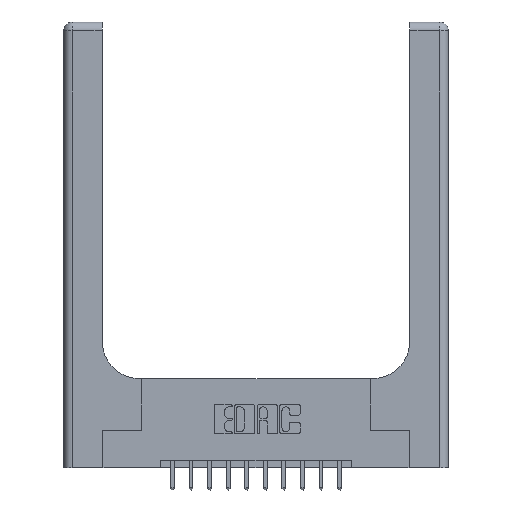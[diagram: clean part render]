
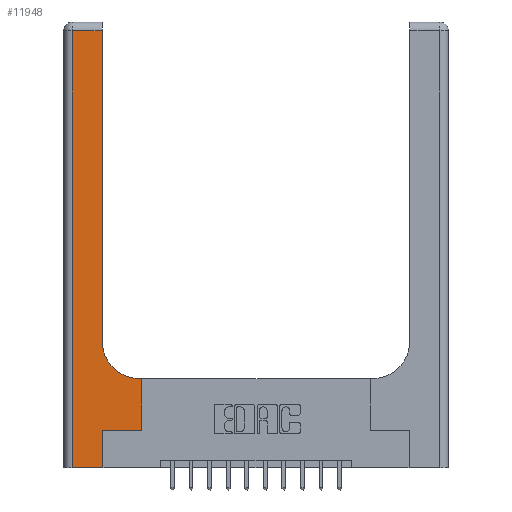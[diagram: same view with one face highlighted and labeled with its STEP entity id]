
A CAD part, top view. The second image highlights one B-rep face of the part: STEP entity #11948.
In plain terms, the highlighted planar face has unit normal (0, 0, 1).
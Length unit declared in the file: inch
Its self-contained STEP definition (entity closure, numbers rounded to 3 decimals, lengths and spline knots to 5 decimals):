
#190 = DIRECTION ( 'NONE',  ( -1., 0., 0. ) ) ;
#330 = VERTEX_POINT ( 'NONE', #12840 ) ;
#437 = CARTESIAN_POINT ( 'NONE',  ( 0.26, 0.6, 0.37 ) ) ;
#578 = EDGE_LOOP ( 'NONE', ( #8681, #5691, #9644, #4940, #738, #8904, #10867, #3484, #5365 ) ) ;
#738 = ORIENTED_EDGE ( 'NONE', *, *, #3867, .T. ) ;
#1101 = EDGE_CURVE ( 'NONE', #2566, #6404, #11632, .T. ) ;
#1329 = DIRECTION ( 'NONE',  ( 1., 0., 0. ) ) ;
#1360 = VERTEX_POINT ( 'NONE', #10355 ) ;
#1429 = CARTESIAN_POINT ( 'NONE',  ( 0.51, 0.85, 0.37 ) ) ;
#2566 = VERTEX_POINT ( 'NONE', #7742 ) ;
#2637 = VECTOR ( 'NONE', #8583, 39.37008 ) ;
#2664 = LINE ( 'NONE', #5162, #10751 ) ;
#2748 = AXIS2_PLACEMENT_3D ( 'NONE', #7198, #4822, #4665 ) ;
#2756 = DIRECTION ( 'NONE',  ( 1., 0., 0. ) ) ;
#2799 = DIRECTION ( 'NONE',  ( 0., 1., 0. ) ) ;
#2901 = DIRECTION ( 'NONE',  ( -1., 0., 0. ) ) ;
#3183 = CARTESIAN_POINT ( 'NONE',  ( 0.51, 0.6, 0.37 ) ) ;
#3458 = AXIS2_PLACEMENT_3D ( 'NONE', #1429, #14357, #2756 ) ;
#3475 = CARTESIAN_POINT ( 'NONE',  ( 0.26, 3., 0.37 ) ) ;
#3484 = ORIENTED_EDGE ( 'NONE', *, *, #1101, .T. ) ;
#3773 = CARTESIAN_POINT ( 'NONE',  ( 0.06, 3., 0.37 ) ) ;
#3837 = VECTOR ( 'NONE', #2901, 39.37008 ) ;
#3867 = EDGE_CURVE ( 'NONE', #11664, #1360, #13060, .T. ) ;
#4095 = VERTEX_POINT ( 'NONE', #4532 ) ;
#4496 = VECTOR ( 'NONE', #2799, 39.37008 ) ;
#4532 = CARTESIAN_POINT ( 'NONE',  ( 0.06, 2.94, 0.37 ) ) ;
#4665 = DIRECTION ( 'NONE',  ( -1., 0., 0. ) ) ;
#4822 = DIRECTION ( 'NONE',  ( 0., 0., -1. ) ) ;
#4940 = ORIENTED_EDGE ( 'NONE', *, *, #7980, .T. ) ;
#5162 = CARTESIAN_POINT ( 'NONE',  ( 0.265, 0.25, 0.37 ) ) ;
#5365 = ORIENTED_EDGE ( 'NONE', *, *, #6035, .T. ) ;
#5516 = EDGE_CURVE ( 'NONE', #4095, #8797, #15300, .T. ) ;
#5691 = ORIENTED_EDGE ( 'NONE', *, *, #15255, .T. ) ;
#5977 = VERTEX_POINT ( 'NONE', #10213 ) ;
#6035 = EDGE_CURVE ( 'NONE', #6404, #5977, #11730, .T. ) ;
#6404 = VERTEX_POINT ( 'NONE', #3183 ) ;
#6464 = VERTEX_POINT ( 'NONE', #8541 ) ;
#6630 = CARTESIAN_POINT ( 'NONE',  ( 0.528, 0.25, 0.37 ) ) ;
#7174 = VECTOR ( 'NONE', #1329, 39.37008 ) ;
#7198 = CARTESIAN_POINT ( 'NONE',  ( 0., 3., 0.37 ) ) ;
#7742 = CARTESIAN_POINT ( 'NONE',  ( 0.528, 0.6, 0.37 ) ) ;
#7810 = VECTOR ( 'NONE', #190, 39.37008 ) ;
#7980 = EDGE_CURVE ( 'NONE', #8797, #11664, #10191, .T. ) ;
#8384 = EDGE_CURVE ( 'NONE', #5977, #330, #11251, .T. ) ;
#8482 = EDGE_CURVE ( 'NONE', #6464, #2566, #9910, .T. ) ;
#8531 = PLANE ( 'NONE',  #2748 ) ;
#8541 = CARTESIAN_POINT ( 'NONE',  ( 0.528, 0.25, 0.37 ) ) ;
#8583 = DIRECTION ( 'NONE',  ( 0., 1., 0. ) ) ;
#8681 = ORIENTED_EDGE ( 'NONE', *, *, #8384, .T. ) ;
#8797 = VERTEX_POINT ( 'NONE', #11621 ) ;
#8904 = ORIENTED_EDGE ( 'NONE', *, *, #13293, .T. ) ;
#9644 = ORIENTED_EDGE ( 'NONE', *, *, #5516, .T. ) ;
#9910 = LINE ( 'NONE', #6630, #12240 ) ;
#10191 = LINE ( 'NONE', #15009, #7174 ) ;
#10213 = CARTESIAN_POINT ( 'NONE',  ( 0.26, 0.85, 0.37 ) ) ;
#10355 = CARTESIAN_POINT ( 'NONE',  ( 0.265, 0.25, 0.37 ) ) ;
#10568 = CARTESIAN_POINT ( 'NONE',  ( 0.265, 0., 0.37 ) ) ;
#10751 = VECTOR ( 'NONE', #11609, 39.37008 ) ;
#10867 = ORIENTED_EDGE ( 'NONE', *, *, #8482, .T. ) ;
#11251 = LINE ( 'NONE', #3475, #2637 ) ;
#11471 = DIRECTION ( 'NONE',  ( 0., -1., 0. ) ) ;
#11609 = DIRECTION ( 'NONE',  ( 1., 0., 0. ) ) ;
#11621 = CARTESIAN_POINT ( 'NONE',  ( 0.06, 0., 0.37 ) ) ;
#11632 = LINE ( 'NONE', #437, #7810 ) ;
#11664 = VERTEX_POINT ( 'NONE', #15442 ) ;
#11730 = CIRCLE ( 'NONE', #3458, 0.25 ) ;
#11948 = ADVANCED_FACE ( 'NONE', ( #12447 ), #8531, .F. ) ;
#12240 = VECTOR ( 'NONE', #16149, 39.37008 ) ;
#12447 = FACE_OUTER_BOUND ( 'NONE', #578, .T. ) ;
#12840 = CARTESIAN_POINT ( 'NONE',  ( 0.26, 2.94, 0.37 ) ) ;
#13060 = LINE ( 'NONE', #10568, #4496 ) ;
#13173 = CARTESIAN_POINT ( 'NONE',  ( 0., 2.94, 0.37 ) ) ;
#13293 = EDGE_CURVE ( 'NONE', #1360, #6464, #2664, .T. ) ;
#14357 = DIRECTION ( 'NONE',  ( 0., 0., -1. ) ) ;
#15009 = CARTESIAN_POINT ( 'NONE',  ( 0., 0., 0.37 ) ) ;
#15157 = VECTOR ( 'NONE', #11471, 39.37008 ) ;
#15255 = EDGE_CURVE ( 'NONE', #330, #4095, #15661, .T. ) ;
#15300 = LINE ( 'NONE', #3773, #15157 ) ;
#15442 = CARTESIAN_POINT ( 'NONE',  ( 0.265, 0., 0.37 ) ) ;
#15661 = LINE ( 'NONE', #13173, #3837 ) ;
#16149 = DIRECTION ( 'NONE',  ( 0., 1., 0. ) ) ;
